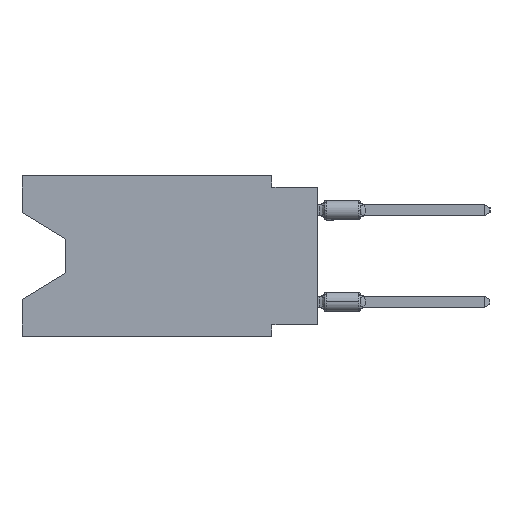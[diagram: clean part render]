
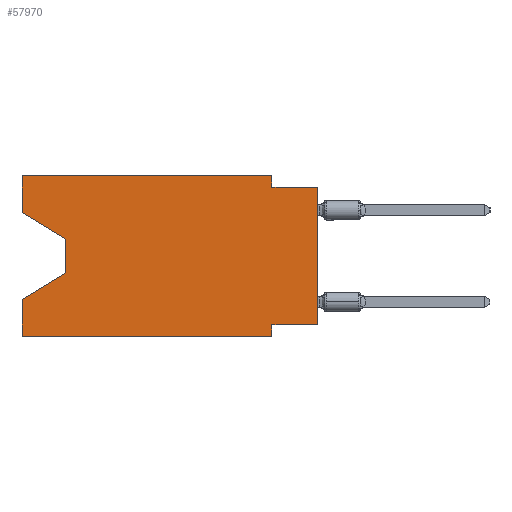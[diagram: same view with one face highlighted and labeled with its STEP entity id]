
A CAD part, left-side view. The second image highlights one B-rep face of the part: STEP entity #57970.
In plain terms, the highlighted planar face has unit normal (-1, 0, 0).
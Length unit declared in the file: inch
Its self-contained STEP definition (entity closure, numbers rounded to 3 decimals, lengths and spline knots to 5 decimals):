
#110 = VECTOR ( 'NONE', #15207, 39.37008 ) ;
#459 = DIRECTION ( 'NONE',  ( 0., 0., 1. ) ) ;
#616 = LINE ( 'NONE', #45106, #11078 ) ;
#2013 = ORIENTED_EDGE ( 'NONE', *, *, #13005, .F. ) ;
#3685 = EDGE_CURVE ( 'NONE', #56043, #38775, #32776, .T. ) ;
#4755 = ORIENTED_EDGE ( 'NONE', *, *, #3685, .T. ) ;
#5719 = EDGE_CURVE ( 'NONE', #26103, #37895, #61254, .T. ) ;
#6083 = LINE ( 'NONE', #41451, #12663 ) ;
#7700 = VERTEX_POINT ( 'NONE', #37725 ) ;
#8086 = CARTESIAN_POINT ( 'NONE',  ( 0., 0., -0.025 ) ) ;
#8117 = DIRECTION ( 'NONE',  ( 0., 0., -1. ) ) ;
#8132 = CARTESIAN_POINT ( 'NONE',  ( 0., 0.645, 0. ) ) ;
#8423 = DIRECTION ( 'NONE',  ( 0., -0.855, -0.519 ) ) ;
#9035 = DIRECTION ( 'NONE',  ( 0., -1., 0. ) ) ;
#9344 = DIRECTION ( 'NONE',  ( 0., -1., 0. ) ) ;
#10718 = ORIENTED_EDGE ( 'NONE', *, *, #60958, .F. ) ;
#10936 = VECTOR ( 'NONE', #9035, 39.37008 ) ;
#11078 = VECTOR ( 'NONE', #55157, 39.37008 ) ;
#12611 = CARTESIAN_POINT ( 'NONE',  ( 0., 0.55, -0.138 ) ) ;
#12663 = VECTOR ( 'NONE', #45062, 39.37008 ) ;
#13005 = EDGE_CURVE ( 'NONE', #46743, #19918, #15524, .T. ) ;
#14228 = CARTESIAN_POINT ( 'NONE',  ( 0., 0., -0.025 ) ) ;
#14863 = ORIENTED_EDGE ( 'NONE', *, *, #29158, .T. ) ;
#15125 = LINE ( 'NONE', #50787, #33294 ) ;
#15207 = DIRECTION ( 'NONE',  ( 0., -1., 0. ) ) ;
#15524 = LINE ( 'NONE', #55090, #110 ) ;
#16401 = CARTESIAN_POINT ( 'NONE',  ( 0., 0.1, -0.35 ) ) ;
#16668 = ORIENTED_EDGE ( 'NONE', *, *, #18420, .F. ) ;
#16935 = PLANE ( 'NONE',  #58121 ) ;
#17264 = DIRECTION ( 'NONE',  ( 1., 0., 0. ) ) ;
#18420 = EDGE_CURVE ( 'NONE', #35011, #38775, #38878, .T. ) ;
#19918 = VERTEX_POINT ( 'NONE', #56369 ) ;
#20543 = EDGE_CURVE ( 'NONE', #19918, #35011, #62306, .T. ) ;
#20628 = LINE ( 'NONE', #30026, #10936 ) ;
#21952 = VECTOR ( 'NONE', #9344, 39.37008 ) ;
#21993 = CARTESIAN_POINT ( 'NONE',  ( 0., 0.55, -0.138 ) ) ;
#22084 = VECTOR ( 'NONE', #8117, 39.37008 ) ;
#23058 = VECTOR ( 'NONE', #27696, 39.37008 ) ;
#26103 = VERTEX_POINT ( 'NONE', #41040 ) ;
#26553 = CARTESIAN_POINT ( 'NONE',  ( 0., 0.55, -0.212 ) ) ;
#26766 = EDGE_CURVE ( 'NONE', #55173, #56522, #57755, .T. ) ;
#27269 = CARTESIAN_POINT ( 'NONE',  ( 0., 0.645, -0.35 ) ) ;
#27696 = DIRECTION ( 'NONE',  ( 0., 0., -1. ) ) ;
#29158 = EDGE_CURVE ( 'NONE', #56522, #26103, #50882, .T. ) ;
#29554 = EDGE_LOOP ( 'NONE', ( #43765, #14863, #48456, #10718, #57521, #47964, #55223, #4755, #16668, #47091, #2013, #53825 ) ) ;
#30026 = CARTESIAN_POINT ( 'NONE',  ( 0., 0.645, -0.35 ) ) ;
#31512 = VECTOR ( 'NONE', #8423, 39.37008 ) ;
#32776 = LINE ( 'NONE', #52573, #51857 ) ;
#33294 = VECTOR ( 'NONE', #459, 39.37008 ) ;
#35011 = VERTEX_POINT ( 'NONE', #46891 ) ;
#37237 = EDGE_CURVE ( 'NONE', #60642, #43707, #20628, .T. ) ;
#37413 = LINE ( 'NONE', #57209, #23058 ) ;
#37647 = CARTESIAN_POINT ( 'NONE',  ( 0., 0.645, -0.08025 ) ) ;
#37665 = FACE_OUTER_BOUND ( 'NONE', #29554, .T. ) ;
#37725 = CARTESIAN_POINT ( 'NONE',  ( 0., 0.1, -0.325 ) ) ;
#37895 = VERTEX_POINT ( 'NONE', #47754 ) ;
#38775 = VERTEX_POINT ( 'NONE', #8086 ) ;
#38878 = LINE ( 'NONE', #14228, #21952 ) ;
#41040 = CARTESIAN_POINT ( 'NONE',  ( 0., 0.55, -0.212 ) ) ;
#41451 = CARTESIAN_POINT ( 'NONE',  ( 0., 0.645, 0. ) ) ;
#41776 = DIRECTION ( 'NONE',  ( 0., 0.855, -0.519 ) ) ;
#41782 = DIRECTION ( 'NONE',  ( 0., 0., -1. ) ) ;
#41864 = DIRECTION ( 'NONE',  ( 0., 0., 1. ) ) ;
#42661 = VECTOR ( 'NONE', #41776, 39.37008 ) ;
#42857 = DIRECTION ( 'NONE',  ( 0., 0., -1. ) ) ;
#43669 = EDGE_CURVE ( 'NONE', #55173, #46743, #15125, .T. ) ;
#43707 = VERTEX_POINT ( 'NONE', #16401 ) ;
#43765 = ORIENTED_EDGE ( 'NONE', *, *, #26766, .T. ) ;
#45062 = DIRECTION ( 'NONE',  ( 0., 0., 1. ) ) ;
#45106 = CARTESIAN_POINT ( 'NONE',  ( 0., 0., -0.325 ) ) ;
#45356 = EDGE_CURVE ( 'NONE', #7700, #43707, #37413, .T. ) ;
#46743 = VERTEX_POINT ( 'NONE', #47658 ) ;
#46891 = CARTESIAN_POINT ( 'NONE',  ( 0., 0.1, -0.025 ) ) ;
#47091 = ORIENTED_EDGE ( 'NONE', *, *, #20543, .F. ) ;
#47398 = CARTESIAN_POINT ( 'NONE',  ( 0., 0., -0.325 ) ) ;
#47658 = CARTESIAN_POINT ( 'NONE',  ( 0., 0.645, 0. ) ) ;
#47754 = CARTESIAN_POINT ( 'NONE',  ( 0., 0.645, -0.26975 ) ) ;
#47964 = ORIENTED_EDGE ( 'NONE', *, *, #45356, .F. ) ;
#48456 = ORIENTED_EDGE ( 'NONE', *, *, #5719, .T. ) ;
#49346 = VECTOR ( 'NONE', #41782, 39.37008 ) ;
#50787 = CARTESIAN_POINT ( 'NONE',  ( 0., 0.645, 0. ) ) ;
#50882 = LINE ( 'NONE', #21993, #49346 ) ;
#51857 = VECTOR ( 'NONE', #41864, 39.37008 ) ;
#52573 = CARTESIAN_POINT ( 'NONE',  ( 0., 0., 0. ) ) ;
#52593 = CARTESIAN_POINT ( 'NONE',  ( 0., 0.1, 0. ) ) ;
#52690 = EDGE_CURVE ( 'NONE', #56043, #7700, #616, .T. ) ;
#53825 = ORIENTED_EDGE ( 'NONE', *, *, #43669, .F. ) ;
#55090 = CARTESIAN_POINT ( 'NONE',  ( 0., 0.645, 0. ) ) ;
#55157 = DIRECTION ( 'NONE',  ( 0., 1., 0. ) ) ;
#55173 = VERTEX_POINT ( 'NONE', #63923 ) ;
#55223 = ORIENTED_EDGE ( 'NONE', *, *, #52690, .F. ) ;
#56043 = VERTEX_POINT ( 'NONE', #47398 ) ;
#56369 = CARTESIAN_POINT ( 'NONE',  ( 0., 0.1, 0. ) ) ;
#56522 = VERTEX_POINT ( 'NONE', #12611 ) ;
#57209 = CARTESIAN_POINT ( 'NONE',  ( 0., 0.1, -0.35 ) ) ;
#57521 = ORIENTED_EDGE ( 'NONE', *, *, #37237, .T. ) ;
#57755 = LINE ( 'NONE', #37647, #31512 ) ;
#57970 = ADVANCED_FACE ( 'NONE', ( #37665 ), #16935, .F. ) ;
#58121 = AXIS2_PLACEMENT_3D ( 'NONE', #8132, #17264, #42857 ) ;
#60642 = VERTEX_POINT ( 'NONE', #27269 ) ;
#60958 = EDGE_CURVE ( 'NONE', #60642, #37895, #6083, .T. ) ;
#61254 = LINE ( 'NONE', #26553, #42661 ) ;
#62306 = LINE ( 'NONE', #52593, #22084 ) ;
#63923 = CARTESIAN_POINT ( 'NONE',  ( 0., 0.645, -0.08025 ) ) ;
